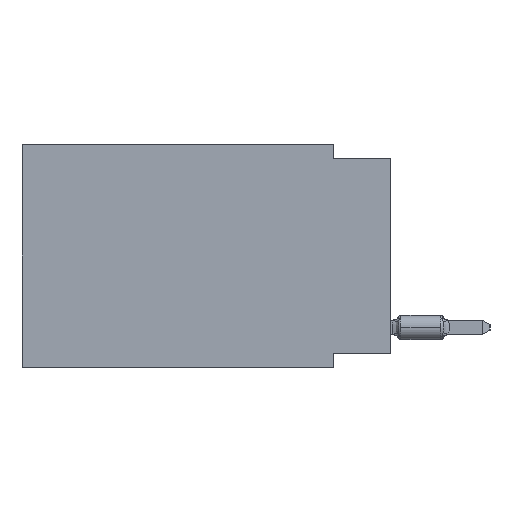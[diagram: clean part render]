
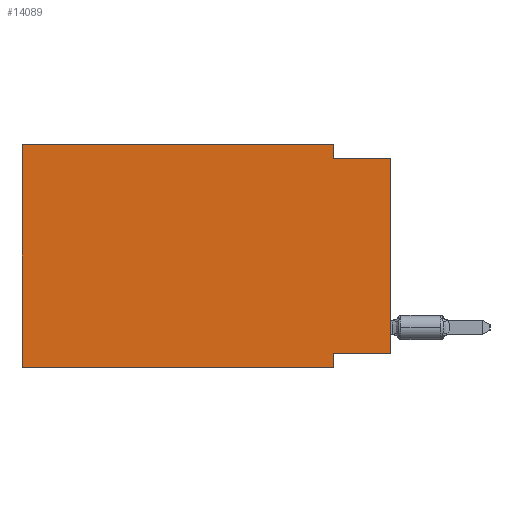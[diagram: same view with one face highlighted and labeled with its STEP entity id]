
A CAD part, left-side view. The second image highlights one B-rep face of the part: STEP entity #14089.
In plain terms, the highlighted planar face has unit normal (-1, 0, 0).
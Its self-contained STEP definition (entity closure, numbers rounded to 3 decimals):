
#229 = CARTESIAN_POINT ( 'NONE',  ( 0., 0., -9.271 ) ) ;
#658 = VECTOR ( 'NONE', #2914, 1000. ) ;
#1251 = VECTOR ( 'NONE', #43374, 1000. ) ;
#1521 = CARTESIAN_POINT ( 'NONE',  ( 0., 0., -9.271 ) ) ;
#2753 = CARTESIAN_POINT ( 'NONE',  ( 0., 2.54, -9.906 ) ) ;
#2840 = ORIENTED_EDGE ( 'NONE', *, *, #23084, .T. ) ;
#2914 = DIRECTION ( 'NONE',  ( 0., 0., 1. ) ) ;
#3084 = CARTESIAN_POINT ( 'NONE',  ( 0., 16.383, 0. ) ) ;
#5387 = ORIENTED_EDGE ( 'NONE', *, *, #21338, .T. ) ;
#5405 = ORIENTED_EDGE ( 'NONE', *, *, #44009, .F. ) ;
#5740 = CARTESIAN_POINT ( 'NONE',  ( 0., 16.383, -9.906 ) ) ;
#5841 = CARTESIAN_POINT ( 'NONE',  ( 0., 0., 0. ) ) ;
#6579 = VECTOR ( 'NONE', #15087, 1000. ) ;
#6728 = ORIENTED_EDGE ( 'NONE', *, *, #37491, .F. ) ;
#7019 = VECTOR ( 'NONE', #39350, 1000. ) ;
#8635 = ORIENTED_EDGE ( 'NONE', *, *, #34070, .F. ) ;
#8769 = CARTESIAN_POINT ( 'NONE',  ( 0., 16.383, 0. ) ) ;
#8785 = VERTEX_POINT ( 'NONE', #28075 ) ;
#9711 = LINE ( 'NONE', #23397, #26718 ) ;
#10244 = CARTESIAN_POINT ( 'NONE',  ( 0., 2.54, -0.635 ) ) ;
#10878 = EDGE_CURVE ( 'NONE', #27983, #24229, #28832, .T. ) ;
#11576 = EDGE_CURVE ( 'NONE', #12364, #22221, #9711, .T. ) ;
#11958 = CARTESIAN_POINT ( 'NONE',  ( 0., 2.54, -9.906 ) ) ;
#12364 = VERTEX_POINT ( 'NONE', #10244 ) ;
#14089 = ADVANCED_FACE ( 'NONE', ( #31302 ), #40936, .F. ) ;
#15087 = DIRECTION ( 'NONE',  ( 0., 0., -1. ) ) ;
#15292 = CARTESIAN_POINT ( 'NONE',  ( 0., 2.54, 0. ) ) ;
#16655 = DIRECTION ( 'NONE',  ( 0., -1., 0. ) ) ;
#17044 = VECTOR ( 'NONE', #28544, 1000. ) ;
#20325 = DIRECTION ( 'NONE',  ( 0., 0., -1. ) ) ;
#21338 = EDGE_CURVE ( 'NONE', #24982, #22221, #43909, .T. ) ;
#22221 = VERTEX_POINT ( 'NONE', #39041 ) ;
#22246 = CARTESIAN_POINT ( 'NONE',  ( 0., 2.54, 0. ) ) ;
#23065 = LINE ( 'NONE', #30233, #658 ) ;
#23084 = EDGE_CURVE ( 'NONE', #43811, #32062, #36414, .T. ) ;
#23397 = CARTESIAN_POINT ( 'NONE',  ( 0., 0., -0.635 ) ) ;
#24229 = VERTEX_POINT ( 'NONE', #15292 ) ;
#24982 = VERTEX_POINT ( 'NONE', #229 ) ;
#25511 = AXIS2_PLACEMENT_3D ( 'NONE', #3084, #40493, #20325 ) ;
#25512 = DIRECTION ( 'NONE',  ( 0., 1., 0. ) ) ;
#26718 = VECTOR ( 'NONE', #16655, 1000. ) ;
#26897 = DIRECTION ( 'NONE',  ( 0., 0., 1. ) ) ;
#27983 = VERTEX_POINT ( 'NONE', #8769 ) ;
#28075 = CARTESIAN_POINT ( 'NONE',  ( 0., 2.54, -9.271 ) ) ;
#28544 = DIRECTION ( 'NONE',  ( 0., 0., -1. ) ) ;
#28751 = ORIENTED_EDGE ( 'NONE', *, *, #37055, .F. ) ;
#28832 = LINE ( 'NONE', #42735, #7019 ) ;
#29290 = ORIENTED_EDGE ( 'NONE', *, *, #10878, .F. ) ;
#30233 = CARTESIAN_POINT ( 'NONE',  ( 0., 16.383, 0. ) ) ;
#31302 = FACE_OUTER_BOUND ( 'NONE', #38518, .T. ) ;
#31872 = VECTOR ( 'NONE', #25512, 1000. ) ;
#32062 = VERTEX_POINT ( 'NONE', #2753 ) ;
#32199 = LINE ( 'NONE', #1521, #31872 ) ;
#34070 = EDGE_CURVE ( 'NONE', #24982, #8785, #32199, .T. ) ;
#35898 = VECTOR ( 'NONE', #26897, 1000. ) ;
#36414 = LINE ( 'NONE', #5740, #1251 ) ;
#37055 = EDGE_CURVE ( 'NONE', #24229, #12364, #42417, .T. ) ;
#37491 = EDGE_CURVE ( 'NONE', #43811, #27983, #23065, .T. ) ;
#38397 = LINE ( 'NONE', #11958, #6579 ) ;
#38518 = EDGE_LOOP ( 'NONE', ( #5387, #39182, #28751, #29290, #6728, #2840, #5405, #8635 ) ) ;
#39041 = CARTESIAN_POINT ( 'NONE',  ( 0., 0., -0.635 ) ) ;
#39182 = ORIENTED_EDGE ( 'NONE', *, *, #11576, .F. ) ;
#39350 = DIRECTION ( 'NONE',  ( 0., -1., 0. ) ) ;
#40493 = DIRECTION ( 'NONE',  ( 1., 0., 0. ) ) ;
#40936 = PLANE ( 'NONE',  #25511 ) ;
#41334 = CARTESIAN_POINT ( 'NONE',  ( 0., 16.383, -9.906 ) ) ;
#42417 = LINE ( 'NONE', #22246, #17044 ) ;
#42735 = CARTESIAN_POINT ( 'NONE',  ( 0., 16.383, 0. ) ) ;
#43374 = DIRECTION ( 'NONE',  ( 0., -1., 0. ) ) ;
#43811 = VERTEX_POINT ( 'NONE', #41334 ) ;
#43909 = LINE ( 'NONE', #5841, #35898 ) ;
#44009 = EDGE_CURVE ( 'NONE', #8785, #32062, #38397, .T. ) ;
